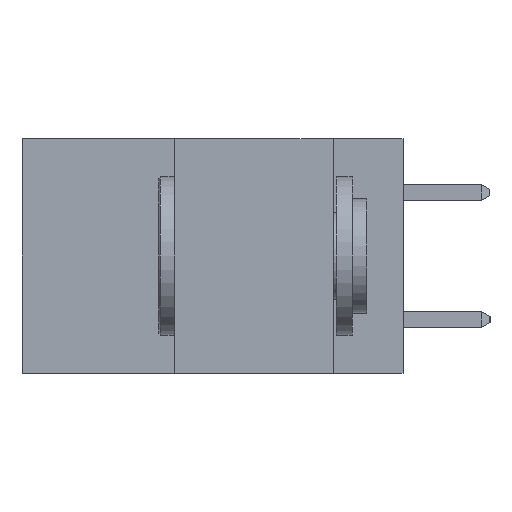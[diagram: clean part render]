
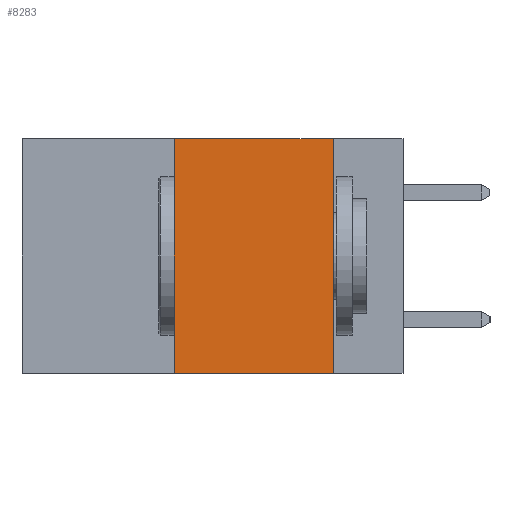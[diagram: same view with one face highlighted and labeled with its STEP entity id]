
A CAD part, left-side view. The second image highlights one B-rep face of the part: STEP entity #8283.
In plain terms, the highlighted planar face has unit normal (-1, 0, 0).
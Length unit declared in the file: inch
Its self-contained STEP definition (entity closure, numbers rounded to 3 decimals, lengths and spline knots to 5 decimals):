
#1511 = CARTESIAN_POINT ( 'NONE',  ( 0., 0.11, -0.37 ) ) ;
#1589 = LINE ( 'NONE', #7494, #8633 ) ;
#2166 = DIRECTION ( 'NONE',  ( 0., -1., 0. ) ) ;
#2618 = LINE ( 'NONE', #11084, #6397 ) ;
#4077 = CARTESIAN_POINT ( 'NONE',  ( 0., 0.36, 0. ) ) ;
#4382 = AXIS2_PLACEMENT_3D ( 'NONE', #9618, #8580, #9665 ) ;
#4450 = VERTEX_POINT ( 'NONE', #7825 ) ;
#4530 = VERTEX_POINT ( 'NONE', #8125 ) ;
#5063 = VERTEX_POINT ( 'NONE', #1511 ) ;
#5432 = DIRECTION ( 'NONE',  ( 0., 0., -1. ) ) ;
#5658 = ORIENTED_EDGE ( 'NONE', *, *, #10079, .F. ) ;
#5910 = DIRECTION ( 'NONE',  ( 0., -1., 0. ) ) ;
#6397 = VECTOR ( 'NONE', #5432, 39.37008 ) ;
#6846 = CARTESIAN_POINT ( 'NONE',  ( 0., 0.36, 0. ) ) ;
#7426 = PLANE ( 'NONE',  #4382 ) ;
#7494 = CARTESIAN_POINT ( 'NONE',  ( 0., 0.6, 0. ) ) ;
#7741 = VERTEX_POINT ( 'NONE', #6846 ) ;
#7825 = CARTESIAN_POINT ( 'NONE',  ( 0., 0.11, 0. ) ) ;
#8125 = CARTESIAN_POINT ( 'NONE',  ( 0., 0.36, -0.37 ) ) ;
#8283 = ADVANCED_FACE ( 'NONE', ( #13378 ), #7426, .F. ) ;
#8391 = EDGE_LOOP ( 'NONE', ( #5658, #11007, #12589, #13342 ) ) ;
#8580 = DIRECTION ( 'NONE',  ( 1., 0., 0. ) ) ;
#8633 = VECTOR ( 'NONE', #2166, 39.37008 ) ;
#9316 = EDGE_CURVE ( 'NONE', #7741, #4450, #1589, .T. ) ;
#9424 = VECTOR ( 'NONE', #12790, 39.37008 ) ;
#9618 = CARTESIAN_POINT ( 'NONE',  ( 0., 0.6, 0. ) ) ;
#9665 = DIRECTION ( 'NONE',  ( 0., 0., -1. ) ) ;
#9859 = EDGE_CURVE ( 'NONE', #4530, #5063, #13331, .T. ) ;
#10079 = EDGE_CURVE ( 'NONE', #4450, #5063, #2618, .T. ) ;
#10384 = VECTOR ( 'NONE', #5910, 39.37008 ) ;
#11007 = ORIENTED_EDGE ( 'NONE', *, *, #9316, .F. ) ;
#11084 = CARTESIAN_POINT ( 'NONE',  ( 0., 0.11, 0. ) ) ;
#11452 = CARTESIAN_POINT ( 'NONE',  ( 0., 0.6, -0.37 ) ) ;
#12589 = ORIENTED_EDGE ( 'NONE', *, *, #13017, .F. ) ;
#12736 = LINE ( 'NONE', #4077, #9424 ) ;
#12790 = DIRECTION ( 'NONE',  ( 0., 0., 1. ) ) ;
#13017 = EDGE_CURVE ( 'NONE', #4530, #7741, #12736, .T. ) ;
#13331 = LINE ( 'NONE', #11452, #10384 ) ;
#13342 = ORIENTED_EDGE ( 'NONE', *, *, #9859, .T. ) ;
#13378 = FACE_OUTER_BOUND ( 'NONE', #8391, .T. ) ;
